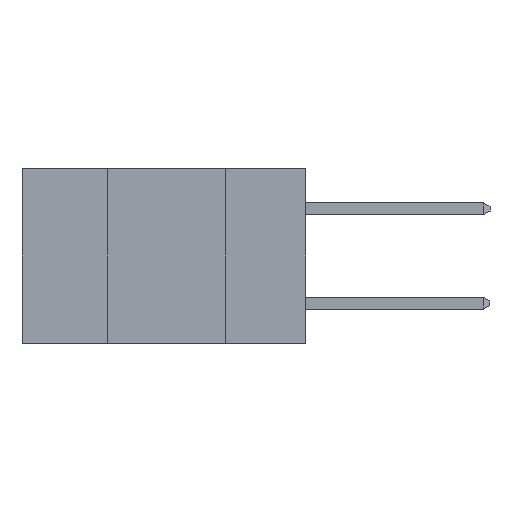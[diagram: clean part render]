
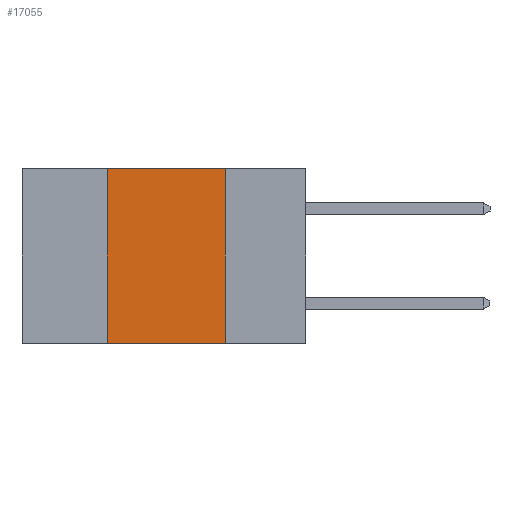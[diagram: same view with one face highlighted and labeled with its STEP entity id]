
A CAD part, left-side view. The second image highlights one B-rep face of the part: STEP entity #17055.
In plain terms, the highlighted planar face has unit normal (-1, 0, 0).
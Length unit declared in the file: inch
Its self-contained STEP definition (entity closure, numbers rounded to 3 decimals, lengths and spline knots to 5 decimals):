
#1257 = AXIS2_PLACEMENT_3D ( 'NONE', #15156, #3894, #19570 ) ;
#2003 = VECTOR ( 'NONE', #9250, 39.37008 ) ;
#2027 = DIRECTION ( 'NONE',  ( 0., -1., 0. ) ) ;
#2531 = EDGE_CURVE ( 'NONE', #12698, #23705, #6344, .T. ) ;
#2538 = CARTESIAN_POINT ( 'NONE',  ( 0., 0.17, 0. ) ) ;
#2980 = DIRECTION ( 'NONE',  ( 0., 0., -1. ) ) ;
#3086 = EDGE_CURVE ( 'NONE', #10792, #23705, #8805, .T. ) ;
#3204 = CARTESIAN_POINT ( 'NONE',  ( 0., 0.17, -0.37 ) ) ;
#3894 = DIRECTION ( 'NONE',  ( 1., 0., 0. ) ) ;
#5624 = VECTOR ( 'NONE', #2980, 39.37008 ) ;
#6344 = LINE ( 'NONE', #2538, #5624 ) ;
#6933 = DIRECTION ( 'NONE',  ( 0., 0., 1. ) ) ;
#8023 = ORIENTED_EDGE ( 'NONE', *, *, #16701, .F. ) ;
#8805 = LINE ( 'NONE', #15887, #2003 ) ;
#9250 = DIRECTION ( 'NONE',  ( 0., -1., 0. ) ) ;
#10118 = VECTOR ( 'NONE', #2027, 39.37008 ) ;
#10792 = VERTEX_POINT ( 'NONE', #13231 ) ;
#12698 = VERTEX_POINT ( 'NONE', #25022 ) ;
#13231 = CARTESIAN_POINT ( 'NONE',  ( 0., 0.42, -0.37 ) ) ;
#15156 = CARTESIAN_POINT ( 'NONE',  ( 0., 0.6, 0. ) ) ;
#15887 = CARTESIAN_POINT ( 'NONE',  ( 0., 0.6, -0.37 ) ) ;
#16701 = EDGE_CURVE ( 'NONE', #10792, #22126, #20972, .T. ) ;
#16747 = LINE ( 'NONE', #28541, #10118 ) ;
#17055 = ADVANCED_FACE ( 'NONE', ( #17219 ), #28137, .F. ) ;
#17219 = FACE_OUTER_BOUND ( 'NONE', #17628, .T. ) ;
#17628 = EDGE_LOOP ( 'NONE', ( #27367, #26552, #8023, #26132 ) ) ;
#19570 = DIRECTION ( 'NONE',  ( 0., 0., -1. ) ) ;
#20316 = VECTOR ( 'NONE', #6933, 39.37008 ) ;
#20972 = LINE ( 'NONE', #22435, #20316 ) ;
#22126 = VERTEX_POINT ( 'NONE', #24803 ) ;
#22435 = CARTESIAN_POINT ( 'NONE',  ( 0., 0.42, 0. ) ) ;
#23317 = EDGE_CURVE ( 'NONE', #22126, #12698, #16747, .T. ) ;
#23705 = VERTEX_POINT ( 'NONE', #3204 ) ;
#24803 = CARTESIAN_POINT ( 'NONE',  ( 0., 0.42, 0. ) ) ;
#25022 = CARTESIAN_POINT ( 'NONE',  ( 0., 0.17, 0. ) ) ;
#26132 = ORIENTED_EDGE ( 'NONE', *, *, #3086, .T. ) ;
#26552 = ORIENTED_EDGE ( 'NONE', *, *, #23317, .F. ) ;
#27367 = ORIENTED_EDGE ( 'NONE', *, *, #2531, .F. ) ;
#28137 = PLANE ( 'NONE',  #1257 ) ;
#28541 = CARTESIAN_POINT ( 'NONE',  ( 0., 0.6, 0. ) ) ;
